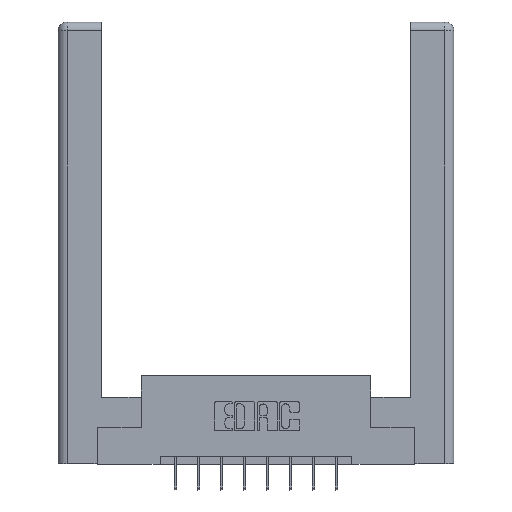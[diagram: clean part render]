
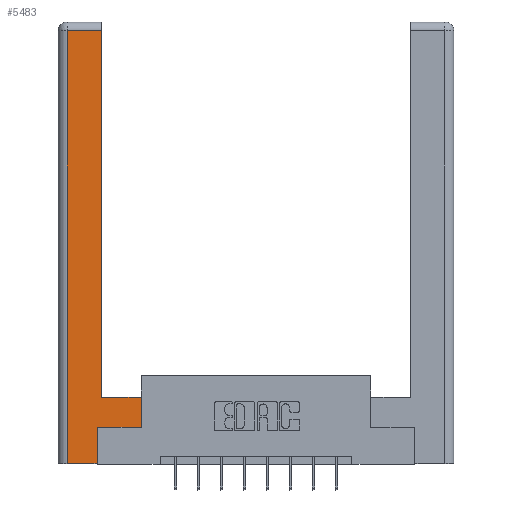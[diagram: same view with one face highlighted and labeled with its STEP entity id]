
A CAD part, top view. The second image highlights one B-rep face of the part: STEP entity #5483.
In plain terms, the highlighted planar face has unit normal (0, 0, 1).
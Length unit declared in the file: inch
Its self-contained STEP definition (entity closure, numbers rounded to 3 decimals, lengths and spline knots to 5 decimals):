
#16 = VERTEX_POINT ( 'NONE', #8326 ) ;
#233 = ORIENTED_EDGE ( 'NONE', *, *, #7956, .T. ) ;
#532 = LINE ( 'NONE', #11667, #13091 ) ;
#1036 = DIRECTION ( 'NONE',  ( 0., 1., 0. ) ) ;
#1232 = EDGE_CURVE ( 'NONE', #8420, #12952, #5076, .T. ) ;
#1553 = VERTEX_POINT ( 'NONE', #1923 ) ;
#1652 = LINE ( 'NONE', #6221, #12319 ) ;
#1923 = CARTESIAN_POINT ( 'NONE',  ( 0.265, 0., 0. ) ) ;
#2255 = LINE ( 'NONE', #9414, #12891 ) ;
#2287 = AXIS2_PLACEMENT_3D ( 'NONE', #11116, #4970, #12146 ) ;
#2415 = CARTESIAN_POINT ( 'NONE',  ( 0.565, 0.245, 0. ) ) ;
#2503 = EDGE_LOOP ( 'NONE', ( #7368, #4172, #5480, #7456, #233, #3666, #9641, #8825 ) ) ;
#2510 = FACE_OUTER_BOUND ( 'NONE', #2503, .T. ) ;
#2638 = CARTESIAN_POINT ( 'NONE',  ( 0.295, 0.45, 0. ) ) ;
#2687 = VECTOR ( 'NONE', #12742, 39.37008 ) ;
#3055 = EDGE_CURVE ( 'NONE', #12952, #1553, #2255, .T. ) ;
#3434 = DIRECTION ( 'NONE',  ( 0., 1., 0. ) ) ;
#3489 = CARTESIAN_POINT ( 'NONE',  ( 0.565, 0.45, 0. ) ) ;
#3666 = ORIENTED_EDGE ( 'NONE', *, *, #5697, .T. ) ;
#3879 = CARTESIAN_POINT ( 'NONE',  ( 0.295, 0.45, 0. ) ) ;
#3995 = LINE ( 'NONE', #8599, #2687 ) ;
#4172 = ORIENTED_EDGE ( 'NONE', *, *, #10355, .T. ) ;
#4406 = VECTOR ( 'NONE', #9863, 39.37008 ) ;
#4970 = DIRECTION ( 'NONE',  ( 0., 0., -1. ) ) ;
#5076 = LINE ( 'NONE', #6535, #11327 ) ;
#5104 = LINE ( 'NONE', #2415, #8639 ) ;
#5301 = VERTEX_POINT ( 'NONE', #3879 ) ;
#5447 = DIRECTION ( 'NONE',  ( 0., -1., 0. ) ) ;
#5480 = ORIENTED_EDGE ( 'NONE', *, *, #1232, .T. ) ;
#5483 = ADVANCED_FACE ( 'NONE', ( #2510 ), #13334, .F. ) ;
#5697 = EDGE_CURVE ( 'NONE', #16, #6663, #5104, .T. ) ;
#6221 = CARTESIAN_POINT ( 'NONE',  ( 0.295, 3., 0. ) ) ;
#6535 = CARTESIAN_POINT ( 'NONE',  ( 0.0615, 0., 0. ) ) ;
#6663 = VERTEX_POINT ( 'NONE', #9172 ) ;
#6702 = VECTOR ( 'NONE', #7048, 39.37008 ) ;
#7048 = DIRECTION ( 'NONE',  ( -1., 0., 0. ) ) ;
#7155 = EDGE_CURVE ( 'NONE', #5301, #10751, #1652, .T. ) ;
#7368 = ORIENTED_EDGE ( 'NONE', *, *, #7155, .T. ) ;
#7453 = VERTEX_POINT ( 'NONE', #3489 ) ;
#7456 = ORIENTED_EDGE ( 'NONE', *, *, #3055, .T. ) ;
#7956 = EDGE_CURVE ( 'NONE', #1553, #16, #3995, .T. ) ;
#8326 = CARTESIAN_POINT ( 'NONE',  ( 0.265, 0.245, 0. ) ) ;
#8420 = VERTEX_POINT ( 'NONE', #12888 ) ;
#8442 = CARTESIAN_POINT ( 'NONE',  ( 0.0615, 0., 0. ) ) ;
#8599 = CARTESIAN_POINT ( 'NONE',  ( 0.265, 0.245, 0. ) ) ;
#8639 = VECTOR ( 'NONE', #12643, 39.37008 ) ;
#8738 = CARTESIAN_POINT ( 'NONE',  ( 0.295, 2.94, 0. ) ) ;
#8825 = ORIENTED_EDGE ( 'NONE', *, *, #11426, .T. ) ;
#9172 = CARTESIAN_POINT ( 'NONE',  ( 0.565, 0.245, 0. ) ) ;
#9414 = CARTESIAN_POINT ( 'NONE',  ( 0.265, 0., 0. ) ) ;
#9641 = ORIENTED_EDGE ( 'NONE', *, *, #10529, .T. ) ;
#9863 = DIRECTION ( 'NONE',  ( -1., 0., 0. ) ) ;
#9876 = LINE ( 'NONE', #2638, #4406 ) ;
#10064 = LINE ( 'NONE', #11146, #6702 ) ;
#10355 = EDGE_CURVE ( 'NONE', #10751, #8420, #10064, .T. ) ;
#10529 = EDGE_CURVE ( 'NONE', #6663, #7453, #532, .T. ) ;
#10751 = VERTEX_POINT ( 'NONE', #8738 ) ;
#11116 = CARTESIAN_POINT ( 'NONE',  ( 0., 0., 0. ) ) ;
#11146 = CARTESIAN_POINT ( 'NONE',  ( 0.0615, 2.94, 0. ) ) ;
#11327 = VECTOR ( 'NONE', #5447, 39.37008 ) ;
#11426 = EDGE_CURVE ( 'NONE', #7453, #5301, #9876, .T. ) ;
#11667 = CARTESIAN_POINT ( 'NONE',  ( 0.565, 0.45, 0. ) ) ;
#12146 = DIRECTION ( 'NONE',  ( -1., 0., 0. ) ) ;
#12319 = VECTOR ( 'NONE', #1036, 39.37008 ) ;
#12575 = DIRECTION ( 'NONE',  ( 1., 0., 0. ) ) ;
#12643 = DIRECTION ( 'NONE',  ( 1., 0., 0. ) ) ;
#12742 = DIRECTION ( 'NONE',  ( 0., 1., 0. ) ) ;
#12888 = CARTESIAN_POINT ( 'NONE',  ( 0.0615, 2.94, 0. ) ) ;
#12891 = VECTOR ( 'NONE', #12575, 39.37008 ) ;
#12952 = VERTEX_POINT ( 'NONE', #8442 ) ;
#13091 = VECTOR ( 'NONE', #3434, 39.37008 ) ;
#13334 = PLANE ( 'NONE',  #2287 ) ;
